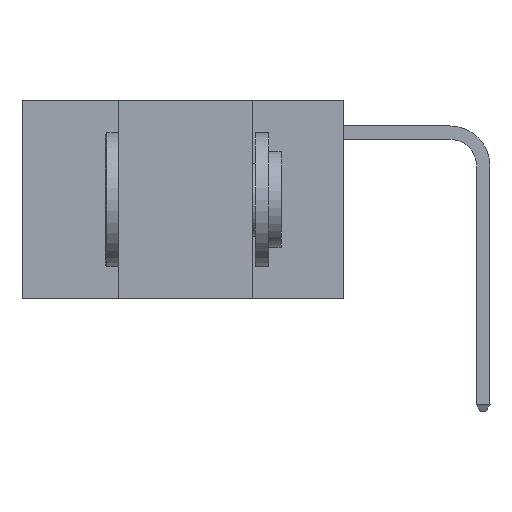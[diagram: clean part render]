
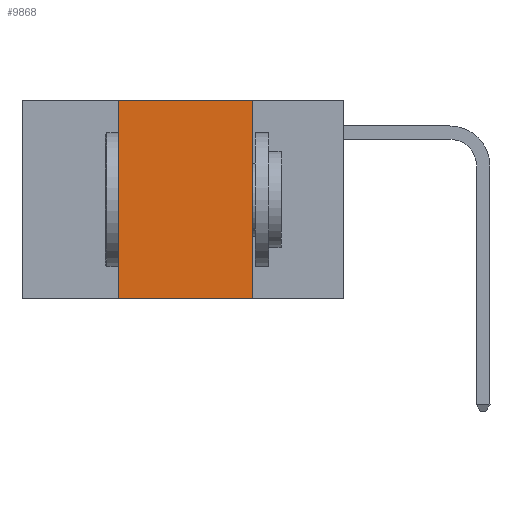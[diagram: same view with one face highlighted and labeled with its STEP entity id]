
A CAD part, left-side view. The second image highlights one B-rep face of the part: STEP entity #9868.
In plain terms, the highlighted planar face has unit normal (-1, 0, 0).
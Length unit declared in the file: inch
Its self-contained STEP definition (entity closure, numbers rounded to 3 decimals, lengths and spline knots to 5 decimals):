
#129 = EDGE_CURVE ( 'NONE', #14365, #14395, #10241, .T. ) ;
#321 = EDGE_CURVE ( 'NONE', #14395, #12892, #1809, .T. ) ;
#720 = ORIENTED_EDGE ( 'NONE', *, *, #7854, .T. ) ;
#1627 = CARTESIAN_POINT ( 'NONE',  ( 0., 0.6, -0.37 ) ) ;
#1809 = LINE ( 'NONE', #15236, #15401 ) ;
#2011 = DIRECTION ( 'NONE',  ( 1., 0., 0. ) ) ;
#2633 = CARTESIAN_POINT ( 'NONE',  ( 0., 0.42, -0.37 ) ) ;
#2819 = CARTESIAN_POINT ( 'NONE',  ( 0., 0.42, 0. ) ) ;
#3528 = ORIENTED_EDGE ( 'NONE', *, *, #4115, .F. ) ;
#4115 = EDGE_CURVE ( 'NONE', #5684, #14365, #4555, .T. ) ;
#4555 = LINE ( 'NONE', #9772, #8918 ) ;
#5355 = DIRECTION ( 'NONE',  ( 0., -1., 0. ) ) ;
#5684 = VERTEX_POINT ( 'NONE', #2633 ) ;
#6580 = EDGE_LOOP ( 'NONE', ( #14488, #9026, #3528, #720 ) ) ;
#7854 = EDGE_CURVE ( 'NONE', #5684, #12892, #8445, .T. ) ;
#8445 = LINE ( 'NONE', #1627, #22151 ) ;
#8918 = VECTOR ( 'NONE', #9406, 39.37008 ) ;
#9026 = ORIENTED_EDGE ( 'NONE', *, *, #129, .F. ) ;
#9381 = PLANE ( 'NONE',  #20428 ) ;
#9406 = DIRECTION ( 'NONE',  ( 0., 0., 1. ) ) ;
#9772 = CARTESIAN_POINT ( 'NONE',  ( 0., 0.42, 0. ) ) ;
#9868 = ADVANCED_FACE ( 'NONE', ( #18586 ), #9381, .F. ) ;
#10241 = LINE ( 'NONE', #17004, #19272 ) ;
#12346 = DIRECTION ( 'NONE',  ( 0., -1., 0. ) ) ;
#12892 = VERTEX_POINT ( 'NONE', #14880 ) ;
#13084 = CARTESIAN_POINT ( 'NONE',  ( 0., 0.6, 0. ) ) ;
#14365 = VERTEX_POINT ( 'NONE', #2819 ) ;
#14395 = VERTEX_POINT ( 'NONE', #23275 ) ;
#14488 = ORIENTED_EDGE ( 'NONE', *, *, #321, .F. ) ;
#14880 = CARTESIAN_POINT ( 'NONE',  ( 0., 0.17, -0.37 ) ) ;
#14914 = DIRECTION ( 'NONE',  ( 0., 0., -1. ) ) ;
#15236 = CARTESIAN_POINT ( 'NONE',  ( 0., 0.17, 0. ) ) ;
#15401 = VECTOR ( 'NONE', #20004, 39.37008 ) ;
#17004 = CARTESIAN_POINT ( 'NONE',  ( 0., 0.6, 0. ) ) ;
#18586 = FACE_OUTER_BOUND ( 'NONE', #6580, .T. ) ;
#19272 = VECTOR ( 'NONE', #12346, 39.37008 ) ;
#20004 = DIRECTION ( 'NONE',  ( 0., 0., -1. ) ) ;
#20428 = AXIS2_PLACEMENT_3D ( 'NONE', #13084, #2011, #14914 ) ;
#22151 = VECTOR ( 'NONE', #5355, 39.37008 ) ;
#23275 = CARTESIAN_POINT ( 'NONE',  ( 0., 0.17, 0. ) ) ;
